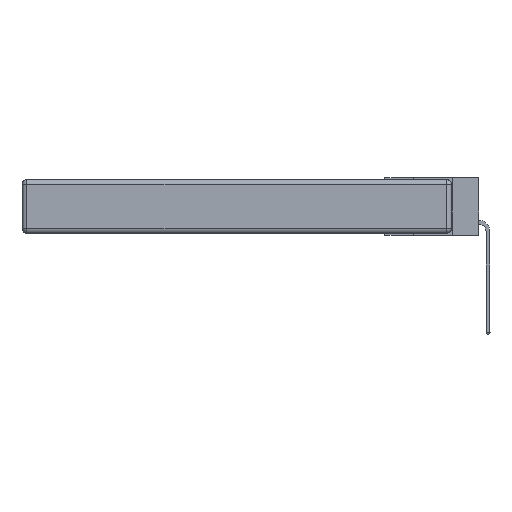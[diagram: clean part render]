
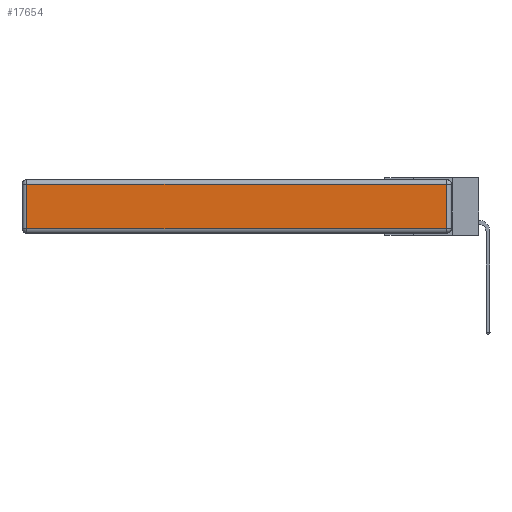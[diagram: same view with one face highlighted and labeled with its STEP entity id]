
A CAD part, left-side view. The second image highlights one B-rep face of the part: STEP entity #17654.
In plain terms, the highlighted planar face has unit normal (-1, 0, 0).
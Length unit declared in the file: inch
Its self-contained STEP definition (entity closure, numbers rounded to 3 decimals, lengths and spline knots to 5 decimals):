
#413 = EDGE_CURVE ( 'NONE', #14122, #2364, #1842, .T. ) ;
#480 = EDGE_LOOP ( 'NONE', ( #8375, #6480, #3166, #19091 ) ) ;
#822 = VECTOR ( 'NONE', #11035, 39.37008 ) ;
#1063 = PLANE ( 'NONE',  #12110 ) ;
#1168 = EDGE_CURVE ( 'NONE', #20254, #14122, #20563, .T. ) ;
#1842 = LINE ( 'NONE', #20320, #10596 ) ;
#2364 = VERTEX_POINT ( 'NONE', #20428 ) ;
#2820 = CARTESIAN_POINT ( 'NONE',  ( 0., 2.72, -0.03 ) ) ;
#2954 = VECTOR ( 'NONE', #7452, 39.37008 ) ;
#3166 = ORIENTED_EDGE ( 'NONE', *, *, #11315, .T. ) ;
#3955 = LINE ( 'NONE', #13511, #10233 ) ;
#4332 = DIRECTION ( 'NONE',  ( 0., 0., 1. ) ) ;
#4397 = CARTESIAN_POINT ( 'NONE',  ( 0., 0., -0.343 ) ) ;
#4755 = EDGE_CURVE ( 'NONE', #2364, #8798, #10985, .T. ) ;
#6212 = CARTESIAN_POINT ( 'NONE',  ( 0., 2.72, -0.343 ) ) ;
#6480 = ORIENTED_EDGE ( 'NONE', *, *, #4755, .T. ) ;
#7452 = DIRECTION ( 'NONE',  ( 0., 0., 1. ) ) ;
#7666 = CARTESIAN_POINT ( 'NONE',  ( 0., 0.03, -0.03 ) ) ;
#8135 = CARTESIAN_POINT ( 'NONE',  ( 0., 2.72, -0.313 ) ) ;
#8375 = ORIENTED_EDGE ( 'NONE', *, *, #413, .T. ) ;
#8798 = VERTEX_POINT ( 'NONE', #7666 ) ;
#10233 = VECTOR ( 'NONE', #13437, 39.37008 ) ;
#10596 = VECTOR ( 'NONE', #16938, 39.37008 ) ;
#10985 = LINE ( 'NONE', #15694, #2954 ) ;
#11035 = DIRECTION ( 'NONE',  ( 0., 0., -1. ) ) ;
#11315 = EDGE_CURVE ( 'NONE', #8798, #20254, #3955, .T. ) ;
#12110 = AXIS2_PLACEMENT_3D ( 'NONE', #4397, #20406, #4332 ) ;
#13437 = DIRECTION ( 'NONE',  ( 0., 1., 0. ) ) ;
#13511 = CARTESIAN_POINT ( 'NONE',  ( 0., 2.75, -0.03 ) ) ;
#14122 = VERTEX_POINT ( 'NONE', #8135 ) ;
#15694 = CARTESIAN_POINT ( 'NONE',  ( 0., 0.03, -0.343 ) ) ;
#15906 = FACE_OUTER_BOUND ( 'NONE', #480, .T. ) ;
#16938 = DIRECTION ( 'NONE',  ( 0., -1., 0. ) ) ;
#17654 = ADVANCED_FACE ( 'NONE', ( #15906 ), #1063, .T. ) ;
#19091 = ORIENTED_EDGE ( 'NONE', *, *, #1168, .T. ) ;
#20254 = VERTEX_POINT ( 'NONE', #2820 ) ;
#20320 = CARTESIAN_POINT ( 'NONE',  ( 0., 0., -0.313 ) ) ;
#20406 = DIRECTION ( 'NONE',  ( -1., 0., 0. ) ) ;
#20428 = CARTESIAN_POINT ( 'NONE',  ( 0., 0.03, -0.313 ) ) ;
#20563 = LINE ( 'NONE', #6212, #822 ) ;
